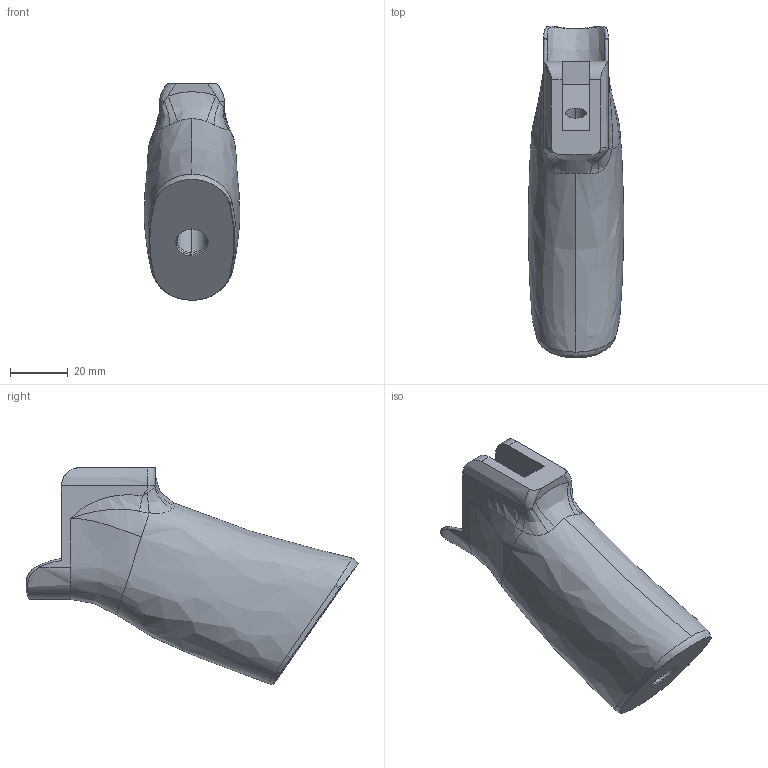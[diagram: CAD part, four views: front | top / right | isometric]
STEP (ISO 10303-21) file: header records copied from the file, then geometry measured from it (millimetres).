
FILE_DESCRIPTION (( 'STEP AP203' ), '1' );
FILE_NAME ('Grip V3.1 Milspec NT.STEP', '2022-05-14T17:19:04', ( '' ), ( '' ), 'SwSTEP 2.0', 'SolidWorks 2021', '' );
FILE_SCHEMA (( 'CONFIG_CONTROL_DESIGN' ));
Length unit declared in the file: inch
Products named in the file (1): Grip V3.1 Milspec NT
Bounding box: 33.2 x 115.21 x 75.18 mm (x, y, z)
Volume: 105559.2 mm3; surface area: 18786.8 mm2
Topology: 1 solids, 1 shells, 63 faces, 170 edges, 107 vertices
Faces by surface type: bspline 42, plane 13, cylinder 8
Entity records: 7768 total; most frequent: CARTESIAN_POINT 6456, ORIENTED_EDGE 332, EDGE_CURVE 166, DIRECTION 138, VERTEX_POINT 107, B_SPLINE_CURVE_WITH_KNOTS 95, EDGE_LOOP 67, ADVANCED_FACE 63
